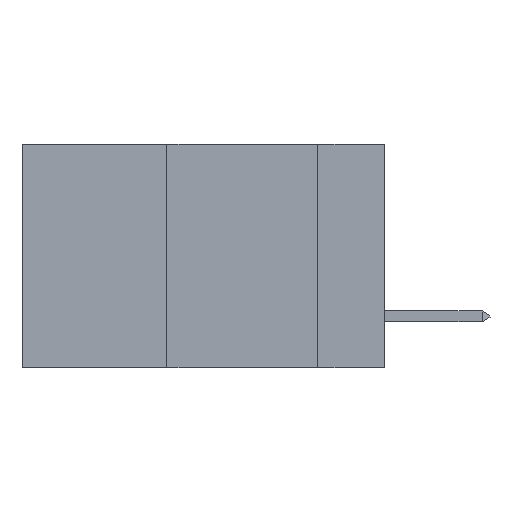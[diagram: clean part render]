
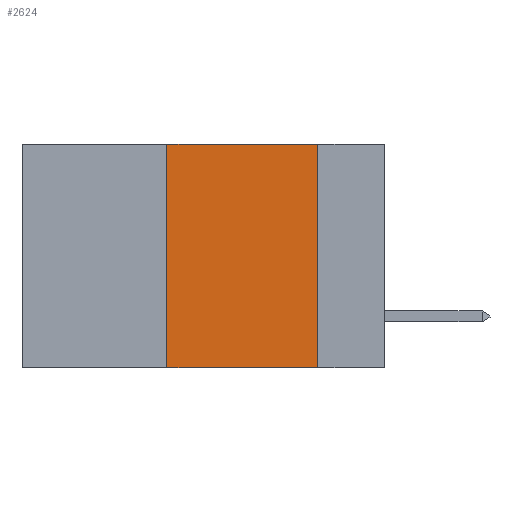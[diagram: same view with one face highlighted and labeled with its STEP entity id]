
A CAD part, left-side view. The second image highlights one B-rep face of the part: STEP entity #2624.
In plain terms, the highlighted planar face has unit normal (-1, 0, 0).
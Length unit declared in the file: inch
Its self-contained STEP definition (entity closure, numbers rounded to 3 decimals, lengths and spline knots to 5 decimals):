
#383 = DIRECTION ( 'NONE',  ( 0., -1., 0. ) ) ;
#1531 = PLANE ( 'NONE',  #20023 ) ;
#2624 = ADVANCED_FACE ( 'NONE', ( #17250 ), #1531, .F. ) ;
#3155 = EDGE_LOOP ( 'NONE', ( #3296, #12040, #7082, #20355 ) ) ;
#3296 = ORIENTED_EDGE ( 'NONE', *, *, #4335, .F. ) ;
#4335 = EDGE_CURVE ( 'NONE', #13110, #6969, #19496, .T. ) ;
#4679 = VERTEX_POINT ( 'NONE', #12451 ) ;
#5100 = CARTESIAN_POINT ( 'NONE',  ( 0., 0.11, 0. ) ) ;
#6185 = VECTOR ( 'NONE', #17582, 39.37008 ) ;
#6969 = VERTEX_POINT ( 'NONE', #10467 ) ;
#7082 = ORIENTED_EDGE ( 'NONE', *, *, #15749, .F. ) ;
#7784 = DIRECTION ( 'NONE',  ( 0., 0., -1. ) ) ;
#7930 = EDGE_CURVE ( 'NONE', #15627, #6969, #19740, .T. ) ;
#9062 = VECTOR ( 'NONE', #20983, 39.37008 ) ;
#9504 = VECTOR ( 'NONE', #7784, 39.37008 ) ;
#9633 = CARTESIAN_POINT ( 'NONE',  ( 0., 0.11, 0. ) ) ;
#9635 = CARTESIAN_POINT ( 'NONE',  ( 0., 0.6, 0. ) ) ;
#10245 = CARTESIAN_POINT ( 'NONE',  ( 0., 0.6, 0. ) ) ;
#10467 = CARTESIAN_POINT ( 'NONE',  ( 0., 0.11, -0.37 ) ) ;
#10640 = EDGE_CURVE ( 'NONE', #4679, #13110, #11407, .T. ) ;
#10996 = CARTESIAN_POINT ( 'NONE',  ( 0., 0.36, -0.37 ) ) ;
#11162 = CARTESIAN_POINT ( 'NONE',  ( 0., 0.6, -0.37 ) ) ;
#11407 = LINE ( 'NONE', #10245, #15552 ) ;
#12040 = ORIENTED_EDGE ( 'NONE', *, *, #10640, .F. ) ;
#12451 = CARTESIAN_POINT ( 'NONE',  ( 0., 0.36, 0. ) ) ;
#12835 = DIRECTION ( 'NONE',  ( 0., 0., -1. ) ) ;
#13110 = VERTEX_POINT ( 'NONE', #5100 ) ;
#14306 = CARTESIAN_POINT ( 'NONE',  ( 0., 0.36, 0. ) ) ;
#15552 = VECTOR ( 'NONE', #383, 39.37008 ) ;
#15627 = VERTEX_POINT ( 'NONE', #10996 ) ;
#15749 = EDGE_CURVE ( 'NONE', #15627, #4679, #17011, .T. ) ;
#16105 = DIRECTION ( 'NONE',  ( 1., 0., 0. ) ) ;
#17011 = LINE ( 'NONE', #14306, #9062 ) ;
#17250 = FACE_OUTER_BOUND ( 'NONE', #3155, .T. ) ;
#17582 = DIRECTION ( 'NONE',  ( 0., -1., 0. ) ) ;
#19496 = LINE ( 'NONE', #9633, #9504 ) ;
#19740 = LINE ( 'NONE', #11162, #6185 ) ;
#20023 = AXIS2_PLACEMENT_3D ( 'NONE', #9635, #16105, #12835 ) ;
#20355 = ORIENTED_EDGE ( 'NONE', *, *, #7930, .T. ) ;
#20983 = DIRECTION ( 'NONE',  ( 0., 0., 1. ) ) ;
